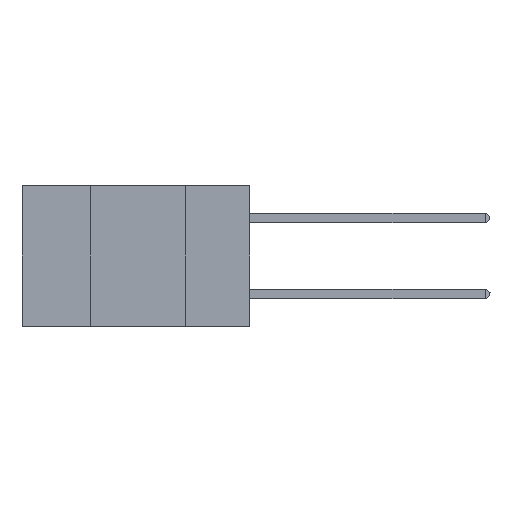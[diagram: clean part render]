
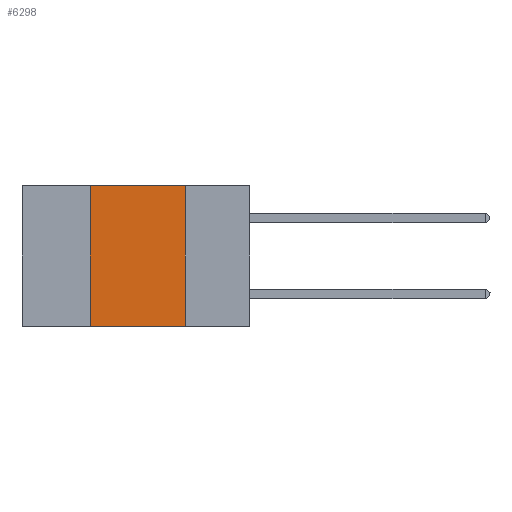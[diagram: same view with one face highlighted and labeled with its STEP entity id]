
A CAD part, left-side view. The second image highlights one B-rep face of the part: STEP entity #6298.
In plain terms, the highlighted planar face has unit normal (-1, 0, 0).
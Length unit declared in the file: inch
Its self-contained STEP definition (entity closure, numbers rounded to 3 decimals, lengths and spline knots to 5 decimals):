
#12 = DIRECTION ( 'NONE',  ( 0., 0., 1. ) ) ;
#1148 = CARTESIAN_POINT ( 'NONE',  ( 0., 0.6, 0. ) ) ;
#1841 = CARTESIAN_POINT ( 'NONE',  ( 0., 0.42, 0. ) ) ;
#2567 = VECTOR ( 'NONE', #19571, 39.37008 ) ;
#2943 = DIRECTION ( 'NONE',  ( 1., 0., 0. ) ) ;
#4023 = VECTOR ( 'NONE', #12, 39.37008 ) ;
#4078 = ORIENTED_EDGE ( 'NONE', *, *, #13441, .F. ) ;
#5704 = EDGE_CURVE ( 'NONE', #19809, #13401, #5996, .T. ) ;
#5996 = LINE ( 'NONE', #9648, #2567 ) ;
#6298 = ADVANCED_FACE ( 'NONE', ( #6567 ), #14530, .F. ) ;
#6567 = FACE_OUTER_BOUND ( 'NONE', #19637, .T. ) ;
#6834 = DIRECTION ( 'NONE',  ( 0., 0., -1. ) ) ;
#6869 = LINE ( 'NONE', #1148, #8036 ) ;
#7853 = EDGE_CURVE ( 'NONE', #15185, #12869, #6869, .T. ) ;
#7971 = LINE ( 'NONE', #15941, #8722 ) ;
#8036 = VECTOR ( 'NONE', #22776, 39.37008 ) ;
#8722 = VECTOR ( 'NONE', #13974, 39.37008 ) ;
#9529 = CARTESIAN_POINT ( 'NONE',  ( 0., 0.17, -0.37 ) ) ;
#9648 = CARTESIAN_POINT ( 'NONE',  ( 0., 0.6, -0.37 ) ) ;
#10543 = CARTESIAN_POINT ( 'NONE',  ( 0., 0.17, 0. ) ) ;
#11576 = ORIENTED_EDGE ( 'NONE', *, *, #7853, .F. ) ;
#12335 = ORIENTED_EDGE ( 'NONE', *, *, #23564, .F. ) ;
#12869 = VERTEX_POINT ( 'NONE', #10543 ) ;
#13401 = VERTEX_POINT ( 'NONE', #9529 ) ;
#13441 = EDGE_CURVE ( 'NONE', #19809, #15185, #19449, .T. ) ;
#13974 = DIRECTION ( 'NONE',  ( 0., 0., -1. ) ) ;
#14530 = PLANE ( 'NONE',  #23793 ) ;
#15185 = VERTEX_POINT ( 'NONE', #23558 ) ;
#15941 = CARTESIAN_POINT ( 'NONE',  ( 0., 0.17, 0. ) ) ;
#16760 = CARTESIAN_POINT ( 'NONE',  ( 0., 0.6, 0. ) ) ;
#19125 = ORIENTED_EDGE ( 'NONE', *, *, #5704, .T. ) ;
#19449 = LINE ( 'NONE', #1841, #4023 ) ;
#19571 = DIRECTION ( 'NONE',  ( 0., -1., 0. ) ) ;
#19637 = EDGE_LOOP ( 'NONE', ( #12335, #11576, #4078, #19125 ) ) ;
#19809 = VERTEX_POINT ( 'NONE', #24559 ) ;
#22776 = DIRECTION ( 'NONE',  ( 0., -1., 0. ) ) ;
#23558 = CARTESIAN_POINT ( 'NONE',  ( 0., 0.42, 0. ) ) ;
#23564 = EDGE_CURVE ( 'NONE', #12869, #13401, #7971, .T. ) ;
#23793 = AXIS2_PLACEMENT_3D ( 'NONE', #16760, #2943, #6834 ) ;
#24559 = CARTESIAN_POINT ( 'NONE',  ( 0., 0.42, -0.37 ) ) ;
